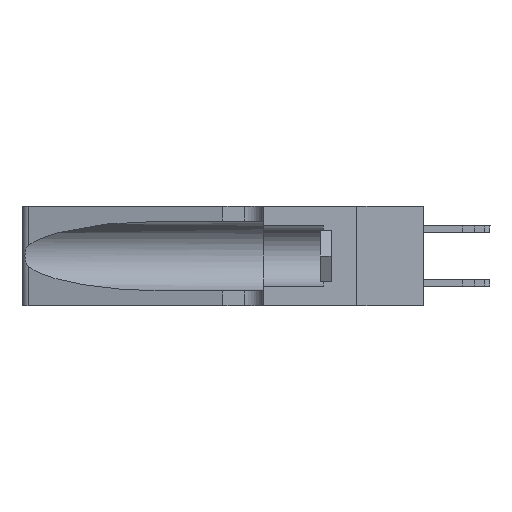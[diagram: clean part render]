
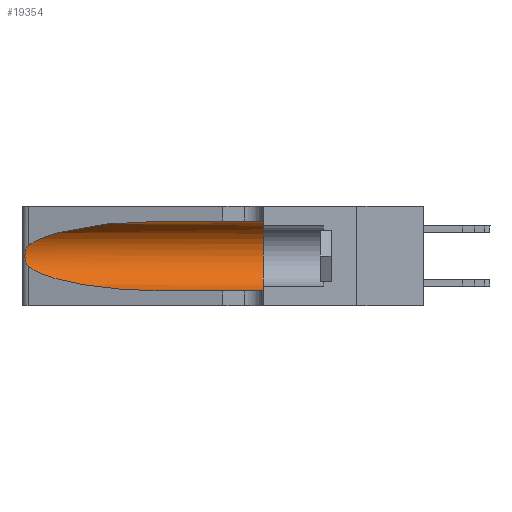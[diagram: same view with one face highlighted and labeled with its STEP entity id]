
A CAD part, left-side view. The second image highlights one B-rep face of the part: STEP entity #19354.
In plain terms, the highlighted cylindrical face has radius 3.308 mm (diameter 6.617 mm), a partial arc.
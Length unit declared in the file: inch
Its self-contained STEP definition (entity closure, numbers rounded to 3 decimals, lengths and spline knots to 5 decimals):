
#322 = CARTESIAN_POINT ( 'NONE',  ( 0.26075, 1.23896, 0.178 ) ) ;
#1395 = CARTESIAN_POINT ( 'NONE',  ( 0.25856, 1.23593, 0.16098 ) ) ;
#1485 = CARTESIAN_POINT ( 'NONE',  ( 0.25555, 1.22993, 0.14849 ) ) ;
#1662 = CARTESIAN_POINT ( 'NONE',  ( 0.25487, 1.22718, 0.14631 ) ) ;
#1736 = CARTESIAN_POINT ( 'NONE',  ( 0.25487, 1.22718, 0.22369 ) ) ;
#3185 = VERTEX_POINT ( 'NONE', #28805 ) ;
#3296 = EDGE_CURVE ( 'NONE', #20692, #3185, #14801, .T. ) ;
#5185 = VERTEX_POINT ( 'NONE', #28582 ) ;
#5343 = ORIENTED_EDGE ( 'NONE', *, *, #8837, .T. ) ;
#5870 = CARTESIAN_POINT ( 'NONE',  ( 0.2373, 1.15595, 0.28018 ) ) ;
#6543 = CARTESIAN_POINT ( 'NONE',  ( 0.1305, 1.61858, 0.31525 ) ) ;
#7264 = CARTESIAN_POINT ( 'NONE',  ( 0.25854, 1.2359, 0.20912 ) ) ;
#8837 = EDGE_CURVE ( 'NONE', #12390, #20692, #22535, .T. ) ;
#8988 = EDGE_LOOP ( 'NONE', ( #22037, #5343, #9961, #26064, #33173, #21273 ) ) ;
#9037 = CARTESIAN_POINT ( 'NONE',  ( 0.25487, 1.22718, 0.14631 ) ) ;
#9204 = DIRECTION ( 'NONE',  ( 0., -1., 0. ) ) ;
#9961 = ORIENTED_EDGE ( 'NONE', *, *, #3296, .T. ) ;
#12390 = VERTEX_POINT ( 'NONE', #1736 ) ;
#14378 =( BOUNDED_CURVE ( )  B_SPLINE_CURVE ( 3, ( #14630, #32166, #5870, #23384 ),
 .UNSPECIFIED., .F., .F. ) 
 B_SPLINE_CURVE_WITH_KNOTS ( ( 4, 4 ),
 ( 1.5708, 2.84003 ),
 .UNSPECIFIED. ) 
 CURVE ( )  GEOMETRIC_REPRESENTATION_ITEM ( )  RATIONAL_B_SPLINE_CURVE ( ( 1., 0.87, 0.87, 1. ) ) 
 REPRESENTATION_ITEM ( '' )  );
#14630 = CARTESIAN_POINT ( 'NONE',  ( 0.1305, 0.72297, 0.31525 ) ) ;
#14801 =( BOUNDED_CURVE ( )  B_SPLINE_CURVE ( 3, ( #9037, #20718, #35584, #14885 ),
 .UNSPECIFIED., .F., .F. ) 
 B_SPLINE_CURVE_WITH_KNOTS ( ( 4, 4 ),
 ( 3.44316, 4.71239 ),
 .UNSPECIFIED. ) 
 CURVE ( )  GEOMETRIC_REPRESENTATION_ITEM ( )  RATIONAL_B_SPLINE_CURVE ( ( 1., 0.87, 0.87, 1. ) ) 
 REPRESENTATION_ITEM ( '' )  );
#14885 = CARTESIAN_POINT ( 'NONE',  ( 0.1305, 0.72297, 0.05475 ) ) ;
#17513 = VERTEX_POINT ( 'NONE', #30200 ) ;
#17583 = VERTEX_POINT ( 'NONE', #33378 ) ;
#18619 = EDGE_CURVE ( 'NONE', #17583, #5185, #33839, .T. ) ;
#19354 = ADVANCED_FACE ( 'NONE', ( #25599 ), #19659, .F. ) ;
#19659 = CYLINDRICAL_SURFACE ( 'NONE', #23179, 0.13025 ) ;
#20011 = AXIS2_PLACEMENT_3D ( 'NONE', #25858, #20212, #23017 ) ;
#20105 = EDGE_CURVE ( 'NONE', #5185, #17513, #28751, .T. ) ;
#20166 = VECTOR ( 'NONE', #24116, 39.37008 ) ;
#20212 = DIRECTION ( 'NONE',  ( 0., 1., 0. ) ) ;
#20304 = CARTESIAN_POINT ( 'NONE',  ( 0.1305, 1.61858, 0.185 ) ) ;
#20692 = VERTEX_POINT ( 'NONE', #21339 ) ;
#20718 = CARTESIAN_POINT ( 'NONE',  ( 0.2373, 1.15595, 0.08982 ) ) ;
#21273 = ORIENTED_EDGE ( 'NONE', *, *, #18619, .F. ) ;
#21339 = CARTESIAN_POINT ( 'NONE',  ( 0.25487, 1.22718, 0.14631 ) ) ;
#22037 = ORIENTED_EDGE ( 'NONE', *, *, #24736, .T. ) ;
#22241 = CARTESIAN_POINT ( 'NONE',  ( 0.25789, 1.23486, 0.15765 ) ) ;
#22535 = B_SPLINE_CURVE_WITH_KNOTS ( 'NONE', 3,
 ( #34516, #22933, #26011, #29543, #7264, #30948, #29247, #322, #34554, #1395, #22241, #24110, #1485, #1662 ),
 .UNSPECIFIED., .F., .F.,
 ( 4, 2, 2, 2, 2, 2, 4 ),
 ( 0., 0.00027, 0.00053, 0.00107, 0.0016, 0.00187, 0.00214 ),
 .UNSPECIFIED. ) ;
#22784 = CARTESIAN_POINT ( 'NONE',  ( 0.1305, 1.61858, 0.05475 ) ) ;
#22933 = CARTESIAN_POINT ( 'NONE',  ( 0.25555, 1.22994, 0.2215 ) ) ;
#23017 = DIRECTION ( 'NONE',  ( 0., 0., 1. ) ) ;
#23179 = AXIS2_PLACEMENT_3D ( 'NONE', #20304, #9204, #27450 ) ;
#23384 = CARTESIAN_POINT ( 'NONE',  ( 0.25487, 1.22718, 0.22369 ) ) ;
#24110 = CARTESIAN_POINT ( 'NONE',  ( 0.25639, 1.23186, 0.15144 ) ) ;
#24116 = DIRECTION ( 'NONE',  ( 0., -1., 0. ) ) ;
#24578 = EDGE_CURVE ( 'NONE', #3185, #17513, #36297, .T. ) ;
#24736 = EDGE_CURVE ( 'NONE', #17583, #12390, #14378, .T. ) ;
#25599 = FACE_OUTER_BOUND ( 'NONE', #8988, .T. ) ;
#25850 = VECTOR ( 'NONE', #31692, 39.37008 ) ;
#25858 = CARTESIAN_POINT ( 'NONE',  ( 0.1305, 0.35, 0.185 ) ) ;
#26011 = CARTESIAN_POINT ( 'NONE',  ( 0.25639, 1.23184, 0.21858 ) ) ;
#26064 = ORIENTED_EDGE ( 'NONE', *, *, #24578, .T. ) ;
#27450 = DIRECTION ( 'NONE',  ( 0., 0., -1. ) ) ;
#28582 = CARTESIAN_POINT ( 'NONE',  ( 0.1305, 0.35, 0.31525 ) ) ;
#28751 = CIRCLE ( 'NONE', #20011, 0.13025 ) ;
#28805 = CARTESIAN_POINT ( 'NONE',  ( 0.1305, 0.72297, 0.05475 ) ) ;
#29247 = CARTESIAN_POINT ( 'NONE',  ( 0.26075, 1.23896, 0.19203 ) ) ;
#29543 = CARTESIAN_POINT ( 'NONE',  ( 0.25787, 1.23484, 0.2124 ) ) ;
#30200 = CARTESIAN_POINT ( 'NONE',  ( 0.1305, 0.35, 0.05475 ) ) ;
#30948 = CARTESIAN_POINT ( 'NONE',  ( 0.26018, 1.23835, 0.19895 ) ) ;
#31692 = DIRECTION ( 'NONE',  ( 0., -1., 0. ) ) ;
#32166 = CARTESIAN_POINT ( 'NONE',  ( 0.18966, 0.96281, 0.31525 ) ) ;
#33173 = ORIENTED_EDGE ( 'NONE', *, *, #20105, .F. ) ;
#33378 = CARTESIAN_POINT ( 'NONE',  ( 0.1305, 0.72297, 0.31525 ) ) ;
#33839 = LINE ( 'NONE', #6543, #20166 ) ;
#34516 = CARTESIAN_POINT ( 'NONE',  ( 0.25487, 1.22718, 0.22369 ) ) ;
#34554 = CARTESIAN_POINT ( 'NONE',  ( 0.26017, 1.23833, 0.17102 ) ) ;
#35584 = CARTESIAN_POINT ( 'NONE',  ( 0.18966, 0.96281, 0.05475 ) ) ;
#36297 = LINE ( 'NONE', #22784, #25850 ) ;
